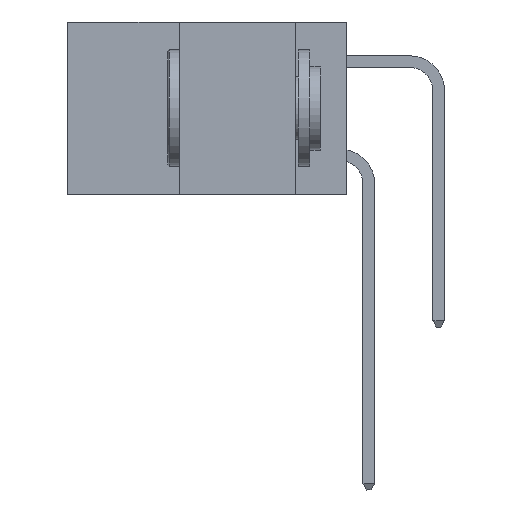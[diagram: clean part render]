
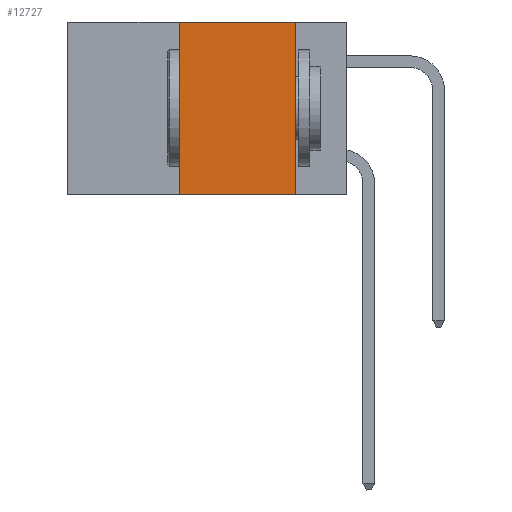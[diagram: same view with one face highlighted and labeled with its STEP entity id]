
A CAD part, left-side view. The second image highlights one B-rep face of the part: STEP entity #12727.
In plain terms, the highlighted planar face has unit normal (-1, 0, 0).
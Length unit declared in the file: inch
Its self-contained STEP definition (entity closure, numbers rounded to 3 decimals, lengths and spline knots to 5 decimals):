
#202 = VERTEX_POINT ( 'NONE', #1580 ) ;
#401 = VERTEX_POINT ( 'NONE', #18507 ) ;
#1039 = VERTEX_POINT ( 'NONE', #8245 ) ;
#1205 = CARTESIAN_POINT ( 'NONE',  ( 0., 0.6, 0. ) ) ;
#1580 = CARTESIAN_POINT ( 'NONE',  ( 0., 0.11, -0.37 ) ) ;
#1717 = EDGE_CURVE ( 'NONE', #401, #12909, #2386, .T. ) ;
#2386 = LINE ( 'NONE', #11864, #16645 ) ;
#2797 = DIRECTION ( 'NONE',  ( 0., 0., -1. ) ) ;
#2975 = DIRECTION ( 'NONE',  ( 0., -1., 0. ) ) ;
#3182 = VECTOR ( 'NONE', #16921, 39.37008 ) ;
#4983 = DIRECTION ( 'NONE',  ( 0., 0., -1. ) ) ;
#5579 = FACE_OUTER_BOUND ( 'NONE', #14784, .T. ) ;
#7298 = EDGE_CURVE ( 'NONE', #1039, #401, #14605, .T. ) ;
#7400 = EDGE_CURVE ( 'NONE', #1039, #202, #16909, .T. ) ;
#7654 = EDGE_CURVE ( 'NONE', #12909, #202, #9896, .T. ) ;
#7699 = CARTESIAN_POINT ( 'NONE',  ( 0., 0.11, 0. ) ) ;
#8245 = CARTESIAN_POINT ( 'NONE',  ( 0., 0.36, -0.37 ) ) ;
#8263 = ORIENTED_EDGE ( 'NONE', *, *, #7400, .T. ) ;
#9057 = ORIENTED_EDGE ( 'NONE', *, *, #7654, .F. ) ;
#9251 = VECTOR ( 'NONE', #2975, 39.37008 ) ;
#9462 = VECTOR ( 'NONE', #4983, 39.37008 ) ;
#9896 = LINE ( 'NONE', #12108, #9462 ) ;
#11545 = DIRECTION ( 'NONE',  ( 1., 0., 0. ) ) ;
#11732 = DIRECTION ( 'NONE',  ( 0., -1., 0. ) ) ;
#11864 = CARTESIAN_POINT ( 'NONE',  ( 0., 0.6, 0. ) ) ;
#12060 = ORIENTED_EDGE ( 'NONE', *, *, #7298, .F. ) ;
#12108 = CARTESIAN_POINT ( 'NONE',  ( 0., 0.11, 0. ) ) ;
#12727 = ADVANCED_FACE ( 'NONE', ( #5579 ), #15623, .F. ) ;
#12829 = CARTESIAN_POINT ( 'NONE',  ( 0., 0.36, 0. ) ) ;
#12909 = VERTEX_POINT ( 'NONE', #7699 ) ;
#14051 = ORIENTED_EDGE ( 'NONE', *, *, #1717, .F. ) ;
#14403 = CARTESIAN_POINT ( 'NONE',  ( 0., 0.6, -0.37 ) ) ;
#14605 = LINE ( 'NONE', #12829, #3182 ) ;
#14784 = EDGE_LOOP ( 'NONE', ( #9057, #14051, #12060, #8263 ) ) ;
#15623 = PLANE ( 'NONE',  #15989 ) ;
#15989 = AXIS2_PLACEMENT_3D ( 'NONE', #1205, #11545, #2797 ) ;
#16645 = VECTOR ( 'NONE', #11732, 39.37008 ) ;
#16909 = LINE ( 'NONE', #14403, #9251 ) ;
#16921 = DIRECTION ( 'NONE',  ( 0., 0., 1. ) ) ;
#18507 = CARTESIAN_POINT ( 'NONE',  ( 0., 0.36, 0. ) ) ;
